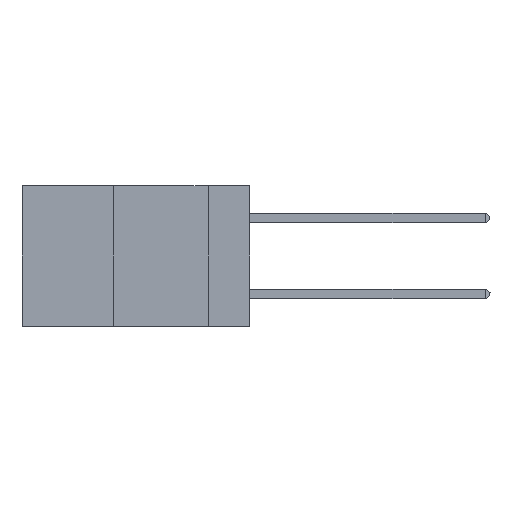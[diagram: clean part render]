
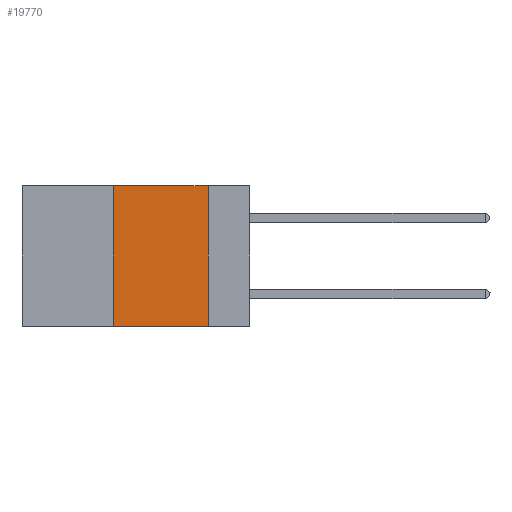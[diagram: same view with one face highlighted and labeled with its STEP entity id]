
A CAD part, left-side view. The second image highlights one B-rep face of the part: STEP entity #19770.
In plain terms, the highlighted planar face has unit normal (-1, 0, 0).
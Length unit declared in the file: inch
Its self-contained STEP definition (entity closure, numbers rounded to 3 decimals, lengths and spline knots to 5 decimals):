
#844 = DIRECTION ( 'NONE',  ( 0., 0., -1. ) ) ;
#2962 = VERTEX_POINT ( 'NONE', #13768 ) ;
#3369 = CARTESIAN_POINT ( 'NONE',  ( 0., 0.6, 0. ) ) ;
#3514 = CARTESIAN_POINT ( 'NONE',  ( 0., 0.6, 0. ) ) ;
#3600 = VECTOR ( 'NONE', #844, 39.37008 ) ;
#4406 = VECTOR ( 'NONE', #6434, 39.37008 ) ;
#5111 = CARTESIAN_POINT ( 'NONE',  ( 0., 0.36, -0.37 ) ) ;
#5240 = CARTESIAN_POINT ( 'NONE',  ( 0., 0.11, 0. ) ) ;
#5316 = VECTOR ( 'NONE', #28349, 39.37008 ) ;
#6178 = CARTESIAN_POINT ( 'NONE',  ( 0., 0.6, -0.37 ) ) ;
#6434 = DIRECTION ( 'NONE',  ( 0., 0., 1. ) ) ;
#7332 = ORIENTED_EDGE ( 'NONE', *, *, #14501, .F. ) ;
#8300 = ORIENTED_EDGE ( 'NONE', *, *, #22864, .F. ) ;
#8802 = ORIENTED_EDGE ( 'NONE', *, *, #14047, .F. ) ;
#9254 = EDGE_CURVE ( 'NONE', #15557, #25792, #26415, .T. ) ;
#10374 = EDGE_LOOP ( 'NONE', ( #7332, #8802, #8300, #11753 ) ) ;
#10392 = DIRECTION ( 'NONE',  ( 0., -1., 0. ) ) ;
#11753 = ORIENTED_EDGE ( 'NONE', *, *, #9254, .T. ) ;
#12449 = LINE ( 'NONE', #3514, #13400 ) ;
#13400 = VECTOR ( 'NONE', #10392, 39.37008 ) ;
#13768 = CARTESIAN_POINT ( 'NONE',  ( 0., 0.36, 0. ) ) ;
#13965 = FACE_OUTER_BOUND ( 'NONE', #10374, .T. ) ;
#14047 = EDGE_CURVE ( 'NONE', #2962, #26483, #12449, .T. ) ;
#14501 = EDGE_CURVE ( 'NONE', #26483, #25792, #27561, .T. ) ;
#15557 = VERTEX_POINT ( 'NONE', #5111 ) ;
#17708 = CARTESIAN_POINT ( 'NONE',  ( 0., 0.36, 0. ) ) ;
#19602 = CARTESIAN_POINT ( 'NONE',  ( 0., 0.11, -0.37 ) ) ;
#19770 = ADVANCED_FACE ( 'NONE', ( #13965 ), #20712, .F. ) ;
#20582 = DIRECTION ( 'NONE',  ( 0., 0., -1. ) ) ;
#20712 = PLANE ( 'NONE',  #22021 ) ;
#22021 = AXIS2_PLACEMENT_3D ( 'NONE', #3369, #23599, #20582 ) ;
#22864 = EDGE_CURVE ( 'NONE', #15557, #2962, #28454, .T. ) ;
#23599 = DIRECTION ( 'NONE',  ( 1., 0., 0. ) ) ;
#25266 = CARTESIAN_POINT ( 'NONE',  ( 0., 0.11, 0. ) ) ;
#25792 = VERTEX_POINT ( 'NONE', #19602 ) ;
#26415 = LINE ( 'NONE', #6178, #5316 ) ;
#26483 = VERTEX_POINT ( 'NONE', #25266 ) ;
#27561 = LINE ( 'NONE', #5240, #3600 ) ;
#28349 = DIRECTION ( 'NONE',  ( 0., -1., 0. ) ) ;
#28454 = LINE ( 'NONE', #17708, #4406 ) ;
